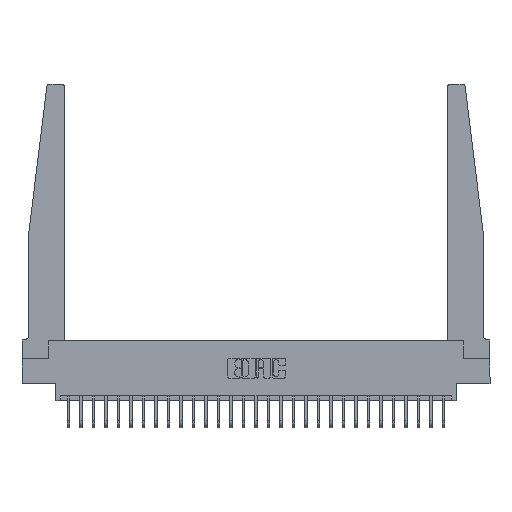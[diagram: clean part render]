
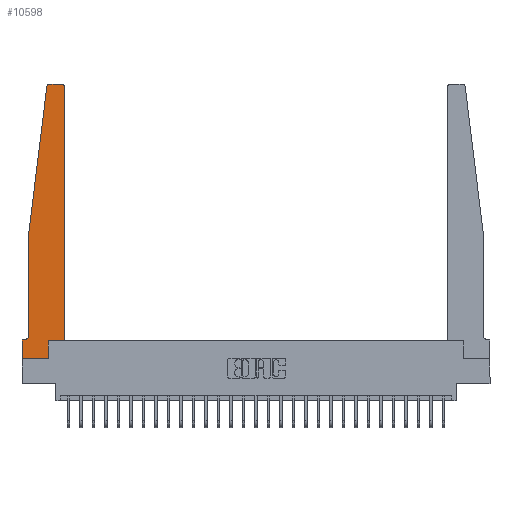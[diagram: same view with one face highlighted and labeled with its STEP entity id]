
A CAD part, top view. The second image highlights one B-rep face of the part: STEP entity #10598.
In plain terms, the highlighted planar face has unit normal (0, 0, 1).
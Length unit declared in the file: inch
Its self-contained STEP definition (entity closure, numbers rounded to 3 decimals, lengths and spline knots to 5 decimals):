
#49 = CARTESIAN_POINT ( 'NONE',  ( 0.065, 0.1875, 0.37 ) ) ;
#105 = DIRECTION ( 'NONE',  ( 0., -1., 0. ) ) ;
#840 = VERTEX_POINT ( 'NONE', #4038 ) ;
#1062 = CARTESIAN_POINT ( 'NONE',  ( 0.015, 0.1875, 0.37 ) ) ;
#1261 = FACE_OUTER_BOUND ( 'NONE', #22191, .T. ) ;
#1564 = VERTEX_POINT ( 'NONE', #16183 ) ;
#1711 = DIRECTION ( 'NONE',  ( -1., 0., 0. ) ) ;
#2275 = CARTESIAN_POINT ( 'NONE',  ( 0.395, 2.75, 0.37 ) ) ;
#3193 = DIRECTION ( 'NONE',  ( 0., 0., 1. ) ) ;
#3942 = EDGE_CURVE ( 'NONE', #24921, #22681, #22065, .T. ) ;
#4038 = CARTESIAN_POINT ( 'NONE',  ( 0.425, 0.18, 0.37 ) ) ;
#4080 = AXIS2_PLACEMENT_3D ( 'NONE', #15868, #26750, #9354 ) ;
#4088 = DIRECTION ( 'NONE',  ( 0., 1., 0. ) ) ;
#4358 = LINE ( 'NONE', #13193, #26682 ) ;
#4733 = CARTESIAN_POINT ( 'NONE',  ( 0.425, 2.72, 0.37 ) ) ;
#4798 = VECTOR ( 'NONE', #4088, 39.37008 ) ;
#4884 = EDGE_CURVE ( 'NONE', #1564, #9367, #10625, .T. ) ;
#5870 = ORIENTED_EDGE ( 'NONE', *, *, #9358, .T. ) ;
#6154 = VERTEX_POINT ( 'NONE', #28005 ) ;
#6218 = ORIENTED_EDGE ( 'NONE', *, *, #27695, .T. ) ;
#6356 = ORIENTED_EDGE ( 'NONE', *, *, #13694, .T. ) ;
#7014 = CARTESIAN_POINT ( 'NONE',  ( 0.065, 1.25, 0.37 ) ) ;
#7171 = CARTESIAN_POINT ( 'NONE',  ( 0.065, 1.25, 0.37 ) ) ;
#7712 = VERTEX_POINT ( 'NONE', #18475 ) ;
#7763 = VECTOR ( 'NONE', #26418, 39.37008 ) ;
#8613 = VECTOR ( 'NONE', #1711, 39.37008 ) ;
#8724 = VECTOR ( 'NONE', #18768, 39.37008 ) ;
#8740 = DIRECTION ( 'NONE',  ( 0., 0., 1. ) ) ;
#9318 = EDGE_CURVE ( 'NONE', #18644, #26230, #17811, .T. ) ;
#9354 = DIRECTION ( 'NONE',  ( 1., 0., 0. ) ) ;
#9358 = EDGE_CURVE ( 'NONE', #6154, #11644, #12305, .T. ) ;
#9367 = VERTEX_POINT ( 'NONE', #15995 ) ;
#9402 = DIRECTION ( 'NONE',  ( 0., 1., 0. ) ) ;
#9527 = ORIENTED_EDGE ( 'NONE', *, *, #9318, .T. ) ;
#9643 = EDGE_CURVE ( 'NONE', #9367, #840, #23596, .T. ) ;
#9771 = CARTESIAN_POINT ( 'NONE',  ( 0., 0., 0.37 ) ) ;
#9786 = ORIENTED_EDGE ( 'NONE', *, *, #18619, .T. ) ;
#10034 = ORIENTED_EDGE ( 'NONE', *, *, #16868, .T. ) ;
#10044 = DIRECTION ( 'NONE',  ( 0., -1., 0. ) ) ;
#10139 = CARTESIAN_POINT ( 'NONE',  ( 0., 0., 0.37 ) ) ;
#10543 = LINE ( 'NONE', #49, #7763 ) ;
#10598 = ADVANCED_FACE ( 'NONE', ( #1261 ), #22578, .T. ) ;
#10625 = LINE ( 'NONE', #18744, #17533 ) ;
#10843 = LINE ( 'NONE', #7014, #26281 ) ;
#10883 = VECTOR ( 'NONE', #12455, 39.37008 ) ;
#11235 = AXIS2_PLACEMENT_3D ( 'NONE', #28050, #8740, #17928 ) ;
#11315 = VECTOR ( 'NONE', #10044, 39.37008 ) ;
#11526 = VERTEX_POINT ( 'NONE', #16857 ) ;
#11644 = VERTEX_POINT ( 'NONE', #13022 ) ;
#12305 = CIRCLE ( 'NONE', #11235, 0.03 ) ;
#12455 = DIRECTION ( 'NONE',  ( 1., 0., 0. ) ) ;
#13022 = CARTESIAN_POINT ( 'NONE',  ( 0.24675, 2.72367, 0.37 ) ) ;
#13193 = CARTESIAN_POINT ( 'NONE',  ( 0.065, 1.25, 0.37 ) ) ;
#13680 = DIRECTION ( 'NONE',  ( -1., 0., 0. ) ) ;
#13694 = EDGE_CURVE ( 'NONE', #26230, #6154, #28218, .T. ) ;
#13806 = DIRECTION ( 'NONE',  ( 1., 0., 0. ) ) ;
#13951 = CARTESIAN_POINT ( 'NONE',  ( 0.015, 0.2375, 0.37 ) ) ;
#14191 = CARTESIAN_POINT ( 'NONE',  ( 0.395, 2.72, 0.37 ) ) ;
#14575 = ORIENTED_EDGE ( 'NONE', *, *, #3942, .T. ) ;
#15228 = EDGE_CURVE ( 'NONE', #7712, #11526, #18920, .T. ) ;
#15868 = CARTESIAN_POINT ( 'NONE',  ( 0., 0.1875, 0.37 ) ) ;
#15887 = DIRECTION ( 'NONE',  ( 0., 0., -1. ) ) ;
#15995 = CARTESIAN_POINT ( 'NONE',  ( 0.2605, 0.18, 0.37 ) ) ;
#16183 = CARTESIAN_POINT ( 'NONE',  ( 0.2605, 0., 0.37 ) ) ;
#16581 = EDGE_CURVE ( 'NONE', #22681, #7712, #10543, .T. ) ;
#16857 = CARTESIAN_POINT ( 'NONE',  ( 0., 0., 0.37 ) ) ;
#16868 = EDGE_CURVE ( 'NONE', #27568, #24921, #4358, .T. ) ;
#16871 = ORIENTED_EDGE ( 'NONE', *, *, #4884, .T. ) ;
#17280 = CARTESIAN_POINT ( 'NONE',  ( 0.425, 0.18, 0.37 ) ) ;
#17533 = VECTOR ( 'NONE', #9402, 39.37008 ) ;
#17811 = CIRCLE ( 'NONE', #27965, 0.03 ) ;
#17928 = DIRECTION ( 'NONE',  ( 1., 0., 0. ) ) ;
#18475 = CARTESIAN_POINT ( 'NONE',  ( 0., 0.1875, 0.37 ) ) ;
#18619 = EDGE_CURVE ( 'NONE', #11644, #27568, #10843, .T. ) ;
#18644 = VERTEX_POINT ( 'NONE', #4733 ) ;
#18744 = CARTESIAN_POINT ( 'NONE',  ( 0.2605, 0.18, 0.37 ) ) ;
#18768 = DIRECTION ( 'NONE',  ( 1., 0., 0. ) ) ;
#18920 = LINE ( 'NONE', #9771, #11315 ) ;
#21665 = EDGE_CURVE ( 'NONE', #840, #18644, #23044, .T. ) ;
#22065 = CIRCLE ( 'NONE', #26202, 0.05 ) ;
#22120 = CARTESIAN_POINT ( 'NONE',  ( 0.065, 0.2375, 0.37 ) ) ;
#22191 = EDGE_LOOP ( 'NONE', ( #6356, #5870, #9786, #10034, #14575, #25637, #23600, #6218, #16871, #23250, #22900, #9527 ) ) ;
#22578 = PLANE ( 'NONE',  #4080 ) ;
#22681 = VERTEX_POINT ( 'NONE', #1062 ) ;
#22900 = ORIENTED_EDGE ( 'NONE', *, *, #21665, .T. ) ;
#23044 = LINE ( 'NONE', #17280, #4798 ) ;
#23250 = ORIENTED_EDGE ( 'NONE', *, *, #9643, .T. ) ;
#23596 = LINE ( 'NONE', #25585, #10883 ) ;
#23600 = ORIENTED_EDGE ( 'NONE', *, *, #15228, .T. ) ;
#24242 = DIRECTION ( 'NONE',  ( -0.122, -0.992, 0. ) ) ;
#24921 = VERTEX_POINT ( 'NONE', #22120 ) ;
#25585 = CARTESIAN_POINT ( 'NONE',  ( 0.425, 0.18, 0.37 ) ) ;
#25637 = ORIENTED_EDGE ( 'NONE', *, *, #16581, .T. ) ;
#25922 = LINE ( 'NONE', #10139, #8724 ) ;
#26202 = AXIS2_PLACEMENT_3D ( 'NONE', #13951, #15887, #13680 ) ;
#26230 = VERTEX_POINT ( 'NONE', #2275 ) ;
#26281 = VECTOR ( 'NONE', #24242, 39.37008 ) ;
#26418 = DIRECTION ( 'NONE',  ( -1., 0., 0. ) ) ;
#26682 = VECTOR ( 'NONE', #105, 39.37008 ) ;
#26750 = DIRECTION ( 'NONE',  ( 0., 0., 1. ) ) ;
#27568 = VERTEX_POINT ( 'NONE', #7171 ) ;
#27695 = EDGE_CURVE ( 'NONE', #11526, #1564, #25922, .T. ) ;
#27965 = AXIS2_PLACEMENT_3D ( 'NONE', #14191, #3193, #13806 ) ;
#27997 = CARTESIAN_POINT ( 'NONE',  ( 0.25, 2.75, 0.37 ) ) ;
#28005 = CARTESIAN_POINT ( 'NONE',  ( 0.27653, 2.75, 0.37 ) ) ;
#28050 = CARTESIAN_POINT ( 'NONE',  ( 0.27653, 2.72, 0.37 ) ) ;
#28218 = LINE ( 'NONE', #27997, #8613 ) ;
